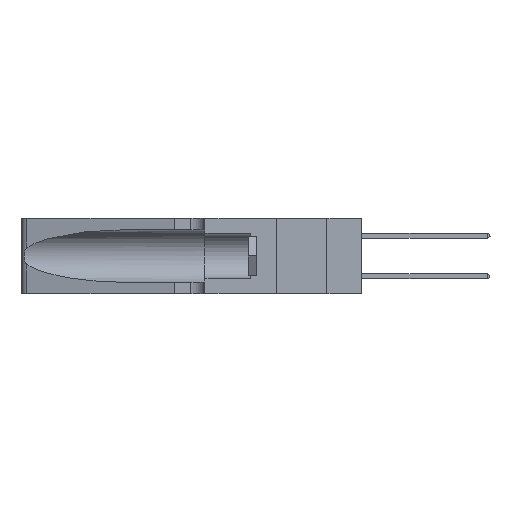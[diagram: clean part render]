
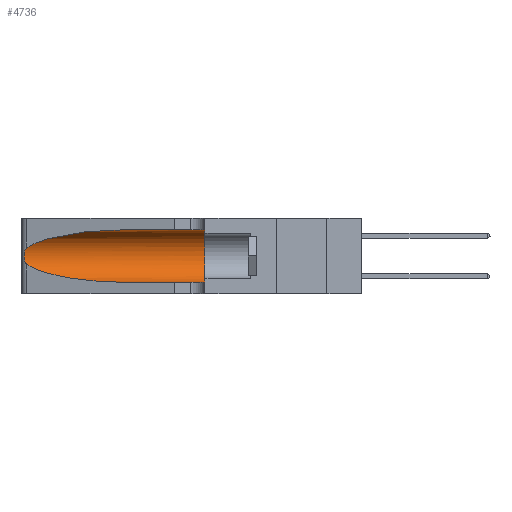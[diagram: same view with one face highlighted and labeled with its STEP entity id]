
A CAD part, left-side view. The second image highlights one B-rep face of the part: STEP entity #4736.
In plain terms, the highlighted cylindrical face has radius 3.308 mm (diameter 6.617 mm), a partial arc.
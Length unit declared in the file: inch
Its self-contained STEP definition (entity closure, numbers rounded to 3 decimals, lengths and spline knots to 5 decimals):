
#989 = EDGE_CURVE ( 'NONE', #12601, #26095, #22275, .T. ) ;
#2728 = CARTESIAN_POINT ( 'NONE',  ( 0.1305, 1.61858, 0.185 ) ) ;
#3170 = DIRECTION ( 'NONE',  ( 0., -1., 0. ) ) ;
#3411 = CARTESIAN_POINT ( 'NONE',  ( 0.26018, 1.23835, 0.19895 ) ) ;
#3613 = EDGE_CURVE ( 'NONE', #36304, #27099, #10964, .T. ) ;
#4586 = CARTESIAN_POINT ( 'NONE',  ( 0.18966, 0.96281, 0.05475 ) ) ;
#4736 = ADVANCED_FACE ( 'NONE', ( #20863 ), #35789, .F. ) ;
#5433 = CARTESIAN_POINT ( 'NONE',  ( 0.26075, 1.23896, 0.178 ) ) ;
#6122 = LINE ( 'NONE', #37549, #7178 ) ;
#7092 = CARTESIAN_POINT ( 'NONE',  ( 0.25787, 1.23484, 0.2124 ) ) ;
#7178 = VECTOR ( 'NONE', #24163, 39.37008 ) ;
#7794 = CARTESIAN_POINT ( 'NONE',  ( 0.1305, 1.61858, 0.31525 ) ) ;
#7892 = AXIS2_PLACEMENT_3D ( 'NONE', #2728, #3170, #34032 ) ;
#9224 = CARTESIAN_POINT ( 'NONE',  ( 0.25487, 1.22718, 0.14631 ) ) ;
#10964 =( BOUNDED_CURVE ( )  B_SPLINE_CURVE ( 3, ( #11969, #15433, #4586, #22369 ),
 .UNSPECIFIED., .F., .T. ) 
 B_SPLINE_CURVE_WITH_KNOTS ( ( 4, 4 ),
 ( 3.44316, 4.71239 ),
 .UNSPECIFIED. ) 
 CURVE ( )  GEOMETRIC_REPRESENTATION_ITEM ( )  RATIONAL_B_SPLINE_CURVE ( ( 1., 0.87, 0.87, 1. ) ) 
 REPRESENTATION_ITEM ( '' )  );
#11073 = CARTESIAN_POINT ( 'NONE',  ( 0.25854, 1.2359, 0.20912 ) ) ;
#11453 = CIRCLE ( 'NONE', #29329, 0.13025 ) ;
#11539 = EDGE_CURVE ( 'NONE', #26095, #36304, #44155, .T. ) ;
#11801 = CARTESIAN_POINT ( 'NONE',  ( 0.1305, 0.72297, 0.05475 ) ) ;
#11969 = CARTESIAN_POINT ( 'NONE',  ( 0.25487, 1.22718, 0.14631 ) ) ;
#12601 = VERTEX_POINT ( 'NONE', #12812 ) ;
#12812 = CARTESIAN_POINT ( 'NONE',  ( 0.1305, 0.72297, 0.31525 ) ) ;
#14358 = CARTESIAN_POINT ( 'NONE',  ( 0.1305, 0.72297, 0.31525 ) ) ;
#14653 = CARTESIAN_POINT ( 'NONE',  ( 0.25487, 1.22718, 0.22369 ) ) ;
#14877 = CARTESIAN_POINT ( 'NONE',  ( 0.25487, 1.22718, 0.22369 ) ) ;
#15076 = CARTESIAN_POINT ( 'NONE',  ( 0.25555, 1.22994, 0.2215 ) ) ;
#15433 = CARTESIAN_POINT ( 'NONE',  ( 0.2373, 1.15595, 0.08982 ) ) ;
#15522 = CARTESIAN_POINT ( 'NONE',  ( 0.25789, 1.23486, 0.15765 ) ) ;
#15910 = ORIENTED_EDGE ( 'NONE', *, *, #33810, .T. ) ;
#15959 = CARTESIAN_POINT ( 'NONE',  ( 0.26075, 1.23896, 0.19203 ) ) ;
#16324 = EDGE_CURVE ( 'NONE', #27833, #41809, #11453, .T. ) ;
#16651 = DIRECTION ( 'NONE',  ( 0., 0., 1. ) ) ;
#19115 = VECTOR ( 'NONE', #28644, 39.37008 ) ;
#20863 = FACE_OUTER_BOUND ( 'NONE', #21623, .T. ) ;
#21623 = EDGE_LOOP ( 'NONE', ( #30731, #42477, #26140, #15910, #41690, #32711 ) ) ;
#21709 = CARTESIAN_POINT ( 'NONE',  ( 0.25487, 1.22718, 0.22369 ) ) ;
#22275 =( BOUNDED_CURVE ( )  B_SPLINE_CURVE ( 3, ( #14358, #35126, #27986, #14653 ),
 .UNSPECIFIED., .F., .F. ) 
 B_SPLINE_CURVE_WITH_KNOTS ( ( 4, 4 ),
 ( 1.5708, 2.84003 ),
 .UNSPECIFIED. ) 
 CURVE ( )  GEOMETRIC_REPRESENTATION_ITEM ( )  RATIONAL_B_SPLINE_CURVE ( ( 1., 0.87, 0.87, 1. ) ) 
 REPRESENTATION_ITEM ( '' )  );
#22369 = CARTESIAN_POINT ( 'NONE',  ( 0.1305, 0.72297, 0.05475 ) ) ;
#23629 = CARTESIAN_POINT ( 'NONE',  ( 0.25487, 1.22718, 0.14631 ) ) ;
#24163 = DIRECTION ( 'NONE',  ( 0., -1., 0. ) ) ;
#26095 = VERTEX_POINT ( 'NONE', #21709 ) ;
#26140 = ORIENTED_EDGE ( 'NONE', *, *, #3613, .T. ) ;
#26450 = CARTESIAN_POINT ( 'NONE',  ( 0.26017, 1.23833, 0.17102 ) ) ;
#26626 = LINE ( 'NONE', #7794, #19115 ) ;
#26799 = CARTESIAN_POINT ( 'NONE',  ( 0.25639, 1.23184, 0.21858 ) ) ;
#26849 = DIRECTION ( 'NONE',  ( 0., 1., 0. ) ) ;
#26998 = CARTESIAN_POINT ( 'NONE',  ( 0.1305, 0.35, 0.185 ) ) ;
#27099 = VERTEX_POINT ( 'NONE', #11801 ) ;
#27833 = VERTEX_POINT ( 'NONE', #43452 ) ;
#27986 = CARTESIAN_POINT ( 'NONE',  ( 0.2373, 1.15595, 0.28018 ) ) ;
#28644 = DIRECTION ( 'NONE',  ( 0., -1., 0. ) ) ;
#29329 = AXIS2_PLACEMENT_3D ( 'NONE', #26998, #26849, #16651 ) ;
#29589 = CARTESIAN_POINT ( 'NONE',  ( 0.25856, 1.23593, 0.16098 ) ) ;
#30731 = ORIENTED_EDGE ( 'NONE', *, *, #989, .T. ) ;
#32711 = ORIENTED_EDGE ( 'NONE', *, *, #33430, .F. ) ;
#33430 = EDGE_CURVE ( 'NONE', #12601, #27833, #26626, .T. ) ;
#33810 = EDGE_CURVE ( 'NONE', #27099, #41809, #6122, .T. ) ;
#34032 = DIRECTION ( 'NONE',  ( 0., 0., -1. ) ) ;
#35126 = CARTESIAN_POINT ( 'NONE',  ( 0.18966, 0.96281, 0.31525 ) ) ;
#35789 = CYLINDRICAL_SURFACE ( 'NONE', #7892, 0.13025 ) ;
#36270 = CARTESIAN_POINT ( 'NONE',  ( 0.25555, 1.22993, 0.14849 ) ) ;
#36304 = VERTEX_POINT ( 'NONE', #23629 ) ;
#37549 = CARTESIAN_POINT ( 'NONE',  ( 0.1305, 1.61858, 0.05475 ) ) ;
#39423 = CARTESIAN_POINT ( 'NONE',  ( 0.25639, 1.23186, 0.15144 ) ) ;
#41247 = CARTESIAN_POINT ( 'NONE',  ( 0.1305, 0.35, 0.05475 ) ) ;
#41690 = ORIENTED_EDGE ( 'NONE', *, *, #16324, .F. ) ;
#41809 = VERTEX_POINT ( 'NONE', #41247 ) ;
#42477 = ORIENTED_EDGE ( 'NONE', *, *, #11539, .T. ) ;
#43452 = CARTESIAN_POINT ( 'NONE',  ( 0.1305, 0.35, 0.31525 ) ) ;
#44155 = B_SPLINE_CURVE_WITH_KNOTS ( 'NONE', 3,
 ( #14877, #15076, #26799, #7092, #11073, #3411, #15959, #5433, #26450, #29589, #15522, #39423, #36270, #9224 ),
 .UNSPECIFIED., .F., .F.,
 ( 4, 2, 2, 2, 2, 2, 4 ),
 ( 0., 0.00027, 0.00053, 0.00107, 0.0016, 0.00187, 0.00214 ),
 .UNSPECIFIED. ) ;
